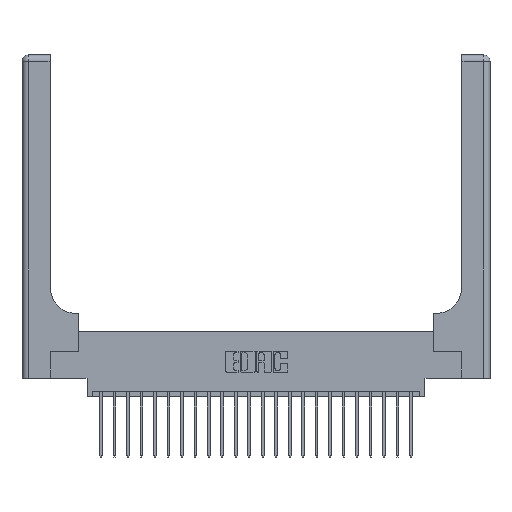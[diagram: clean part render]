
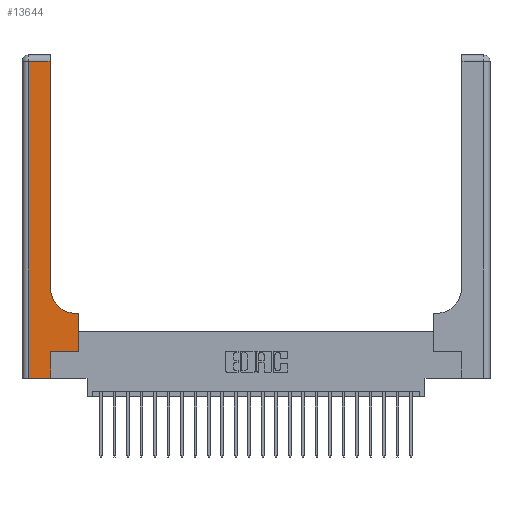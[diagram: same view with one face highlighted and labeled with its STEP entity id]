
A CAD part, top view. The second image highlights one B-rep face of the part: STEP entity #13644.
In plain terms, the highlighted planar face has unit normal (0, 0, 1).
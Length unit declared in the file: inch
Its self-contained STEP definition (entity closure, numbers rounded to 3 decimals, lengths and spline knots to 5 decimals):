
#922 = DIRECTION ( 'NONE',  ( 0., 1., 0. ) ) ;
#1470 = VECTOR ( 'NONE', #16551, 39.37008 ) ;
#1587 = VERTEX_POINT ( 'NONE', #6724 ) ;
#1735 = CARTESIAN_POINT ( 'NONE',  ( 0.265, 0.25, 0.37 ) ) ;
#2014 = VERTEX_POINT ( 'NONE', #6578 ) ;
#2273 = CARTESIAN_POINT ( 'NONE',  ( 0., 2.94, 0.37 ) ) ;
#2799 = CARTESIAN_POINT ( 'NONE',  ( 0., 3., 0.37 ) ) ;
#4281 = ORIENTED_EDGE ( 'NONE', *, *, #7572, .T. ) ;
#4418 = ORIENTED_EDGE ( 'NONE', *, *, #10319, .T. ) ;
#5210 = VECTOR ( 'NONE', #5353, 39.37008 ) ;
#5353 = DIRECTION ( 'NONE',  ( 0., -1., 0. ) ) ;
#6125 = DIRECTION ( 'NONE',  ( 1., 0., 0. ) ) ;
#6398 = CIRCLE ( 'NONE', #12563, 0.25 ) ;
#6578 = CARTESIAN_POINT ( 'NONE',  ( 0.26, 0.85, 0.37 ) ) ;
#6724 = CARTESIAN_POINT ( 'NONE',  ( 0.51, 0.6, 0.37 ) ) ;
#7497 = ORIENTED_EDGE ( 'NONE', *, *, #17863, .T. ) ;
#7530 = VERTEX_POINT ( 'NONE', #23604 ) ;
#7543 = CARTESIAN_POINT ( 'NONE',  ( 0.528, 0.25, 0.37 ) ) ;
#7572 = EDGE_CURVE ( 'NONE', #7530, #16989, #18299, .T. ) ;
#8113 = DIRECTION ( 'NONE',  ( 1., 0., 0. ) ) ;
#8400 = EDGE_CURVE ( 'NONE', #23858, #18191, #21615, .T. ) ;
#8472 = VECTOR ( 'NONE', #922, 39.37008 ) ;
#8552 = CARTESIAN_POINT ( 'NONE',  ( 0.26, 3., 0.37 ) ) ;
#9108 = DIRECTION ( 'NONE',  ( 1., 0., 0. ) ) ;
#9288 = LINE ( 'NONE', #2273, #1470 ) ;
#9612 = CARTESIAN_POINT ( 'NONE',  ( 0.528, 0.6, 0.37 ) ) ;
#9645 = CARTESIAN_POINT ( 'NONE',  ( 0.26, 2.94, 0.37 ) ) ;
#9740 = CARTESIAN_POINT ( 'NONE',  ( 0.06, 2.94, 0.37 ) ) ;
#9918 = CARTESIAN_POINT ( 'NONE',  ( 0.51, 0.85, 0.37 ) ) ;
#10319 = EDGE_CURVE ( 'NONE', #18191, #7530, #17600, .T. ) ;
#10894 = CARTESIAN_POINT ( 'NONE',  ( 0.06, 3., 0.37 ) ) ;
#11084 = EDGE_CURVE ( 'NONE', #2014, #16646, #19671, .T. ) ;
#11196 = CARTESIAN_POINT ( 'NONE',  ( 0.528, 0.25, 0.37 ) ) ;
#11227 = ORIENTED_EDGE ( 'NONE', *, *, #13375, .T. ) ;
#11288 = LINE ( 'NONE', #7543, #19937 ) ;
#11474 = CARTESIAN_POINT ( 'NONE',  ( 0.06, 0., 0.37 ) ) ;
#11657 = EDGE_CURVE ( 'NONE', #16989, #17007, #11288, .T. ) ;
#11798 = CARTESIAN_POINT ( 'NONE',  ( 0.265, 0., 0.37 ) ) ;
#11895 = ORIENTED_EDGE ( 'NONE', *, *, #11084, .T. ) ;
#12285 = EDGE_LOOP ( 'NONE', ( #11895, #22938, #11227, #16576, #4418, #4281, #13599, #7497, #14844 ) ) ;
#12365 = LINE ( 'NONE', #10894, #5210 ) ;
#12563 = AXIS2_PLACEMENT_3D ( 'NONE', #9918, #17309, #8113 ) ;
#13185 = VERTEX_POINT ( 'NONE', #9740 ) ;
#13302 = CARTESIAN_POINT ( 'NONE',  ( 0.26, 0.6, 0.37 ) ) ;
#13375 = EDGE_CURVE ( 'NONE', #13185, #23858, #12365, .T. ) ;
#13564 = FACE_OUTER_BOUND ( 'NONE', #12285, .T. ) ;
#13599 = ORIENTED_EDGE ( 'NONE', *, *, #11657, .T. ) ;
#13644 = ADVANCED_FACE ( 'NONE', ( #13564 ), #15251, .F. ) ;
#13674 = DIRECTION ( 'NONE',  ( -1., 0., 0. ) ) ;
#13704 = EDGE_CURVE ( 'NONE', #1587, #2014, #6398, .T. ) ;
#13726 = CARTESIAN_POINT ( 'NONE',  ( 0., 0., 0.37 ) ) ;
#14844 = ORIENTED_EDGE ( 'NONE', *, *, #13704, .T. ) ;
#14923 = DIRECTION ( 'NONE',  ( 0., 1., 0. ) ) ;
#15251 = PLANE ( 'NONE',  #16057 ) ;
#16057 = AXIS2_PLACEMENT_3D ( 'NONE', #2799, #22589, #13674 ) ;
#16325 = CARTESIAN_POINT ( 'NONE',  ( 0.265, 0., 0.37 ) ) ;
#16551 = DIRECTION ( 'NONE',  ( -1., 0., 0. ) ) ;
#16576 = ORIENTED_EDGE ( 'NONE', *, *, #8400, .T. ) ;
#16646 = VERTEX_POINT ( 'NONE', #9645 ) ;
#16989 = VERTEX_POINT ( 'NONE', #11196 ) ;
#17007 = VERTEX_POINT ( 'NONE', #9612 ) ;
#17309 = DIRECTION ( 'NONE',  ( 0., 0., -1. ) ) ;
#17589 = VECTOR ( 'NONE', #18384, 39.37008 ) ;
#17600 = LINE ( 'NONE', #11798, #8472 ) ;
#17680 = VECTOR ( 'NONE', #9108, 39.37008 ) ;
#17863 = EDGE_CURVE ( 'NONE', #17007, #1587, #20185, .T. ) ;
#18014 = VECTOR ( 'NONE', #6125, 39.37008 ) ;
#18191 = VERTEX_POINT ( 'NONE', #16325 ) ;
#18299 = LINE ( 'NONE', #1735, #17680 ) ;
#18384 = DIRECTION ( 'NONE',  ( -1., 0., 0. ) ) ;
#19433 = DIRECTION ( 'NONE',  ( 0., 1., 0. ) ) ;
#19671 = LINE ( 'NONE', #8552, #20685 ) ;
#19937 = VECTOR ( 'NONE', #14923, 39.37008 ) ;
#20185 = LINE ( 'NONE', #13302, #17589 ) ;
#20685 = VECTOR ( 'NONE', #19433, 39.37008 ) ;
#21615 = LINE ( 'NONE', #13726, #18014 ) ;
#22589 = DIRECTION ( 'NONE',  ( 0., 0., -1. ) ) ;
#22772 = EDGE_CURVE ( 'NONE', #16646, #13185, #9288, .T. ) ;
#22938 = ORIENTED_EDGE ( 'NONE', *, *, #22772, .T. ) ;
#23604 = CARTESIAN_POINT ( 'NONE',  ( 0.265, 0.25, 0.37 ) ) ;
#23858 = VERTEX_POINT ( 'NONE', #11474 ) ;
